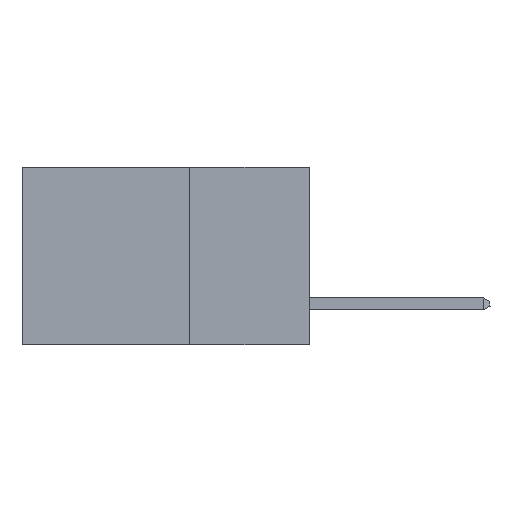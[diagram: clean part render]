
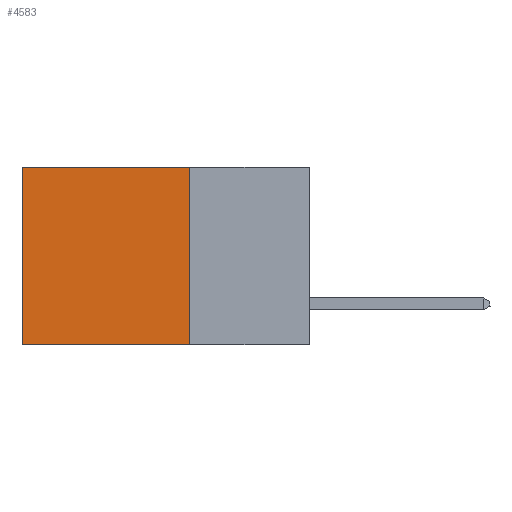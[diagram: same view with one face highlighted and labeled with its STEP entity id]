
A CAD part, left-side view. The second image highlights one B-rep face of the part: STEP entity #4583.
In plain terms, the highlighted planar face has unit normal (-1, 0, 0).
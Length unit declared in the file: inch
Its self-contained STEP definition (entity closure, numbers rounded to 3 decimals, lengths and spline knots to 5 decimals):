
#680 = ORIENTED_EDGE ( 'NONE', *, *, #19466, .T. ) ;
#869 = ORIENTED_EDGE ( 'NONE', *, *, #31195, .T. ) ;
#1046 = DIRECTION ( 'NONE',  ( 0., 0., -1. ) ) ;
#1851 = VERTEX_POINT ( 'NONE', #2757 ) ;
#2757 = CARTESIAN_POINT ( 'NONE',  ( 0.2875, 0.6, 0. ) ) ;
#3091 = ORIENTED_EDGE ( 'NONE', *, *, #35973, .F. ) ;
#4547 = FACE_OUTER_BOUND ( 'NONE', #9315, .T. ) ;
#4583 = ADVANCED_FACE ( 'NONE', ( #4547 ), #10147, .F. ) ;
#5097 = VECTOR ( 'NONE', #32871, 39.37008 ) ;
#5645 = EDGE_CURVE ( 'NONE', #21734, #37704, #14251, .T. ) ;
#7240 = CARTESIAN_POINT ( 'NONE',  ( 0.2875, 0.25, 0. ) ) ;
#8006 = CARTESIAN_POINT ( 'NONE',  ( 0.2875, 0.25, 0. ) ) ;
#9315 = EDGE_LOOP ( 'NONE', ( #680, #26140, #3091, #869 ) ) ;
#9621 = DIRECTION ( 'NONE',  ( 0., 0., -1. ) ) ;
#9642 = DIRECTION ( 'NONE',  ( 0., 1., 0. ) ) ;
#9972 = CARTESIAN_POINT ( 'NONE',  ( 0.2875, 0.25, -0.37 ) ) ;
#10147 = PLANE ( 'NONE',  #26672 ) ;
#11545 = CARTESIAN_POINT ( 'NONE',  ( 0.2875, 0.25, 0. ) ) ;
#13614 = CARTESIAN_POINT ( 'NONE',  ( 0.2875, 0.6, -0.37 ) ) ;
#14251 = LINE ( 'NONE', #38074, #26115 ) ;
#16242 = VECTOR ( 'NONE', #21058, 39.37008 ) ;
#17378 = CARTESIAN_POINT ( 'NONE',  ( 0.2875, 0.25, 0. ) ) ;
#17445 = VECTOR ( 'NONE', #9621, 39.37008 ) ;
#19466 = EDGE_CURVE ( 'NONE', #1851, #37704, #25386, .T. ) ;
#21058 = DIRECTION ( 'NONE',  ( 0., 0., -1. ) ) ;
#21734 = VERTEX_POINT ( 'NONE', #9972 ) ;
#25386 = LINE ( 'NONE', #34591, #17445 ) ;
#26115 = VECTOR ( 'NONE', #9642, 39.37008 ) ;
#26140 = ORIENTED_EDGE ( 'NONE', *, *, #5645, .F. ) ;
#26158 = LINE ( 'NONE', #11545, #16242 ) ;
#26672 = AXIS2_PLACEMENT_3D ( 'NONE', #7240, #35787, #1046 ) ;
#28260 = LINE ( 'NONE', #8006, #5097 ) ;
#31195 = EDGE_CURVE ( 'NONE', #33463, #1851, #28260, .T. ) ;
#32871 = DIRECTION ( 'NONE',  ( 0., 1., 0. ) ) ;
#33463 = VERTEX_POINT ( 'NONE', #17378 ) ;
#34591 = CARTESIAN_POINT ( 'NONE',  ( 0.2875, 0.6, 0. ) ) ;
#35787 = DIRECTION ( 'NONE',  ( 1., 0., 0. ) ) ;
#35973 = EDGE_CURVE ( 'NONE', #33463, #21734, #26158, .T. ) ;
#37704 = VERTEX_POINT ( 'NONE', #13614 ) ;
#38074 = CARTESIAN_POINT ( 'NONE',  ( 0.2875, 0.25, -0.37 ) ) ;
